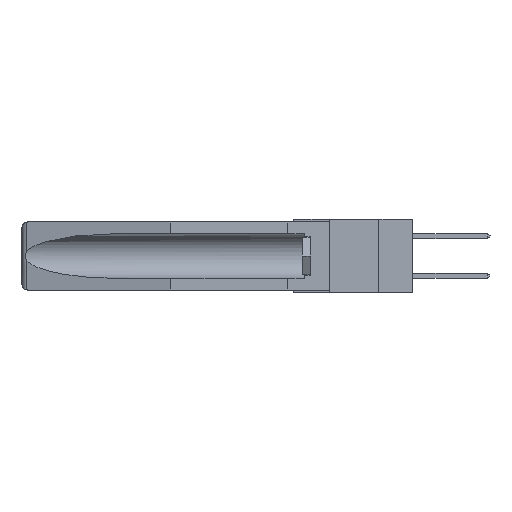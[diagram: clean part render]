
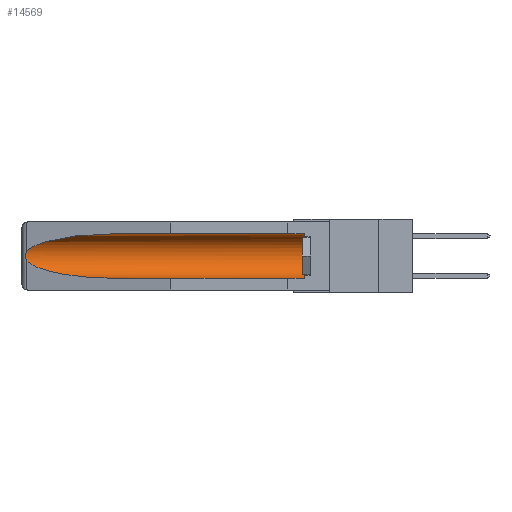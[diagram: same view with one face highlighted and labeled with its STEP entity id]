
A CAD part, left-side view. The second image highlights one B-rep face of the part: STEP entity #14569.
In plain terms, the highlighted cylindrical face has radius 2.857 mm (diameter 5.715 mm), a partial arc.
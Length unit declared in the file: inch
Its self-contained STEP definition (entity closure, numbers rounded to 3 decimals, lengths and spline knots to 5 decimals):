
#185 = CARTESIAN_POINT ( 'NONE',  ( 0.155, -0.30754, -0.059 ) ) ;
#719 = EDGE_CURVE ( 'NONE', #22498, #12769, #22143, .T. ) ;
#1091 = CARTESIAN_POINT ( 'NONE',  ( 0.155, -0.30754, -0.284 ) ) ;
#1209 = CARTESIAN_POINT ( 'NONE',  ( 0.26597, 1.52961, -0.15275 ) ) ;
#1224 = ORIENTED_EDGE ( 'NONE', *, *, #719, .T. ) ;
#1228 = CARTESIAN_POINT ( 'NONE',  ( 0.26537, 1.52718, -0.14972 ) ) ;
#1294 = CARTESIAN_POINT ( 'NONE',  ( 0.26537, 1.52718, -0.19328 ) ) ;
#2165 = CIRCLE ( 'NONE', #24496, 0.1125 ) ;
#2400 = VERTEX_POINT ( 'NONE', #9296 ) ;
#2417 = EDGE_CURVE ( 'NONE', #23944, #22498, #17270, .T. ) ;
#2592 = DIRECTION ( 'NONE',  ( 0., 1., 0. ) ) ;
#2809 = FACE_OUTER_BOUND ( 'NONE', #5035, .T. ) ;
#2950 = DIRECTION ( 'NONE',  ( 0., 1., 0. ) ) ;
#3213 = CARTESIAN_POINT ( 'NONE',  ( 0.155, 0.126, -0.1715 ) ) ;
#3449 = VERTEX_POINT ( 'NONE', #21215 ) ;
#3575 = CARTESIAN_POINT ( 'NONE',  ( 0.155, 1.07973, -0.059 ) ) ;
#4153 = CYLINDRICAL_SURFACE ( 'NONE', #23397, 0.1125 ) ;
#5035 = EDGE_LOOP ( 'NONE', ( #24097, #1224, #6826, #16788, #16587, #10146 ) ) ;
#5168 = EDGE_CURVE ( 'NONE', #2400, #3449, #2165, .T. ) ;
#5418 = DIRECTION ( 'NONE',  ( 0., -1., 0. ) ) ;
#5455 = CARTESIAN_POINT ( 'NONE',  ( 0.2673, 1.53269, -0.17917 ) ) ;
#5873 = VECTOR ( 'NONE', #2950, 39.37008 ) ;
#6826 = ORIENTED_EDGE ( 'NONE', *, *, #25686, .T. ) ;
#6829 = CARTESIAN_POINT ( 'NONE',  ( 0.21114, 1.30732, -0.059 ) ) ;
#7426 = CARTESIAN_POINT ( 'NONE',  ( 0.26654, 1.53092, -0.15636 ) ) ;
#7559 = DIRECTION ( 'NONE',  ( 0., 0., 1. ) ) ;
#9152 = VECTOR ( 'NONE', #10863, 39.37008 ) ;
#9296 = CARTESIAN_POINT ( 'NONE',  ( 0.155, 0.126, -0.284 ) ) ;
#9889 = LINE ( 'NONE', #1091, #5873 ) ;
#10146 = ORIENTED_EDGE ( 'NONE', *, *, #13549, .T. ) ;
#10863 = DIRECTION ( 'NONE',  ( 0., 1., 0. ) ) ;
#11020 = CARTESIAN_POINT ( 'NONE',  ( 0.26537, 1.52718, -0.19328 ) ) ;
#11203 = CARTESIAN_POINT ( 'NONE',  ( 0.25451, 1.48313, -0.24835 ) ) ;
#11587 = VERTEX_POINT ( 'NONE', #21948 ) ;
#12769 = VERTEX_POINT ( 'NONE', #24344 ) ;
#13147 = EDGE_CURVE ( 'NONE', #2400, #11587, #9889, .T. ) ;
#13160 = CARTESIAN_POINT ( 'NONE',  ( 0.21114, 1.30732, -0.284 ) ) ;
#13260 = DIRECTION ( 'NONE',  ( 0., 0., 1. ) ) ;
#13549 = EDGE_CURVE ( 'NONE', #3449, #23944, #26721, .T. ) ;
#14569 = ADVANCED_FACE ( 'NONE', ( #2809 ), #4153, .F. ) ;
#15082 = CARTESIAN_POINT ( 'NONE',  ( 0.25451, 1.48313, -0.09465 ) ) ;
#15304 = CARTESIAN_POINT ( 'NONE',  ( 0.155, -0.30754, -0.1715 ) ) ;
#16161 = CARTESIAN_POINT ( 'NONE',  ( 0.26537, 1.52718, -0.14972 ) ) ;
#16587 = ORIENTED_EDGE ( 'NONE', *, *, #5168, .T. ) ;
#16788 = ORIENTED_EDGE ( 'NONE', *, *, #13147, .F. ) ;
#17270 =( BOUNDED_CURVE ( )  B_SPLINE_CURVE ( 3, ( #19176, #6829, #15082, #17427 ),
 .UNSPECIFIED., .F., .F. ) 
 B_SPLINE_CURVE_WITH_KNOTS ( ( 4, 4 ),
 ( 4.71239, 6.08839 ),
 .UNSPECIFIED. ) 
 CURVE ( )  GEOMETRIC_REPRESENTATION_ITEM ( )  RATIONAL_B_SPLINE_CURVE ( ( 1., 0.848, 0.848, 1. ) ) 
 REPRESENTATION_ITEM ( '' )  );
#17427 = CARTESIAN_POINT ( 'NONE',  ( 0.26537, 1.52718, -0.14972 ) ) ;
#17523 = CARTESIAN_POINT ( 'NONE',  ( 0.155, 1.07973, -0.284 ) ) ;
#18002 = CARTESIAN_POINT ( 'NONE',  ( 0.2673, 1.5327, -0.16383 ) ) ;
#18721 =( BOUNDED_CURVE ( )  B_SPLINE_CURVE ( 3, ( #11020, #11203, #13160, #17523 ),
 .UNSPECIFIED., .F., .F. ) 
 B_SPLINE_CURVE_WITH_KNOTS ( ( 4, 4 ),
 ( 0.1948, 1.5708 ),
 .UNSPECIFIED. ) 
 CURVE ( )  GEOMETRIC_REPRESENTATION_ITEM ( )  RATIONAL_B_SPLINE_CURVE ( ( 1., 0.848, 0.848, 1. ) ) 
 REPRESENTATION_ITEM ( '' )  );
#19176 = CARTESIAN_POINT ( 'NONE',  ( 0.155, 1.07973, -0.059 ) ) ;
#20018 = CARTESIAN_POINT ( 'NONE',  ( 0.2675, 1.53308, -0.16763 ) ) ;
#20193 = CARTESIAN_POINT ( 'NONE',  ( 0.26655, 1.53094, -0.18657 ) ) ;
#21215 = CARTESIAN_POINT ( 'NONE',  ( 0.155, 0.126, -0.059 ) ) ;
#21948 = CARTESIAN_POINT ( 'NONE',  ( 0.155, 1.07973, -0.284 ) ) ;
#22143 = B_SPLINE_CURVE_WITH_KNOTS ( 'NONE', 3,
 ( #16161, #1209, #7426, #18002, #20018, #24335, #5455, #20193, #22309, #1294 ),
 .UNSPECIFIED., .F., .F.,
 ( 4, 2, 2, 2, 4 ),
 ( 0., 0.00029, 0.00058, 0.00087, 0.00117 ),
 .UNSPECIFIED. ) ;
#22309 = CARTESIAN_POINT ( 'NONE',  ( 0.26597, 1.5296, -0.19026 ) ) ;
#22498 = VERTEX_POINT ( 'NONE', #1228 ) ;
#23397 = AXIS2_PLACEMENT_3D ( 'NONE', #15304, #2592, #13260 ) ;
#23944 = VERTEX_POINT ( 'NONE', #3575 ) ;
#24097 = ORIENTED_EDGE ( 'NONE', *, *, #2417, .T. ) ;
#24335 = CARTESIAN_POINT ( 'NONE',  ( 0.2675, 1.53308, -0.17534 ) ) ;
#24344 = CARTESIAN_POINT ( 'NONE',  ( 0.26537, 1.52718, -0.19328 ) ) ;
#24496 = AXIS2_PLACEMENT_3D ( 'NONE', #3213, #5418, #7559 ) ;
#25686 = EDGE_CURVE ( 'NONE', #12769, #11587, #18721, .T. ) ;
#26721 = LINE ( 'NONE', #185, #9152 ) ;
